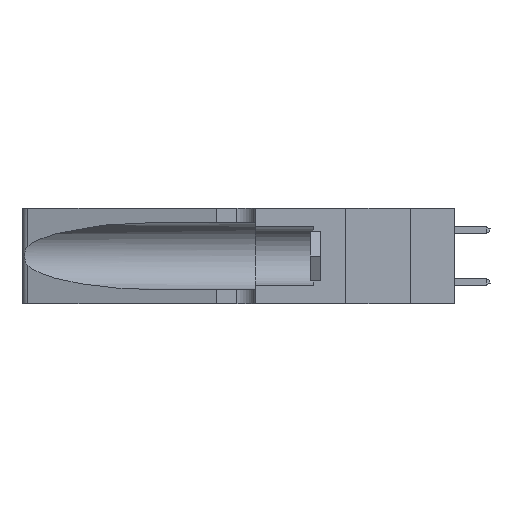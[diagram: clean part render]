
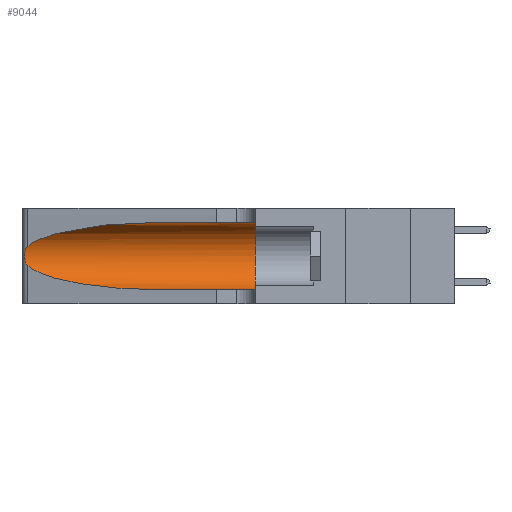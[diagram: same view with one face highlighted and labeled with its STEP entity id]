
A CAD part, left-side view. The second image highlights one B-rep face of the part: STEP entity #9044.
In plain terms, the highlighted cylindrical face has radius 3.308 mm (diameter 6.617 mm), a partial arc.
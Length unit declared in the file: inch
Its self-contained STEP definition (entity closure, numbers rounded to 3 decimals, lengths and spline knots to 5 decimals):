
#729 = VERTEX_POINT ( 'NONE', #15652 ) ;
#792 = EDGE_CURVE ( 'NONE', #729, #7416, #15196, .T. ) ;
#983 = CARTESIAN_POINT ( 'NONE',  ( 0.1305, 0.35, 0.31525 ) ) ;
#1715 = CARTESIAN_POINT ( 'NONE',  ( 0.1305, 0.35, 0.185 ) ) ;
#2022 = CARTESIAN_POINT ( 'NONE',  ( 0.1305, 1.61858, 0.185 ) ) ;
#2512 = VECTOR ( 'NONE', #16649, 39.37008 ) ;
#3192 = CARTESIAN_POINT ( 'NONE',  ( 0.2373, 1.15595, 0.28018 ) ) ;
#3324 = CARTESIAN_POINT ( 'NONE',  ( 0.25487, 1.22718, 0.14631 ) ) ;
#3396 = VERTEX_POINT ( 'NONE', #24382 ) ;
#3710 = DIRECTION ( 'NONE',  ( 0., 0., 1. ) ) ;
#4066 = ORIENTED_EDGE ( 'NONE', *, *, #13687, .F. ) ;
#4930 = CARTESIAN_POINT ( 'NONE',  ( 0.1305, 0.72297, 0.05475 ) ) ;
#5242 = EDGE_CURVE ( 'NONE', #3396, #14820, #7758, .T. ) ;
#5308 = CARTESIAN_POINT ( 'NONE',  ( 0.2373, 1.15595, 0.08982 ) ) ;
#6062 = EDGE_CURVE ( 'NONE', #10185, #8558, #24668, .T. ) ;
#6814 = AXIS2_PLACEMENT_3D ( 'NONE', #2022, #19379, #11790 ) ;
#7270 = CARTESIAN_POINT ( 'NONE',  ( 0.18966, 0.96281, 0.05475 ) ) ;
#7416 = VERTEX_POINT ( 'NONE', #22352 ) ;
#7457 = EDGE_CURVE ( 'NONE', #7416, #10185, #17749, .T. ) ;
#7758 = LINE ( 'NONE', #22335, #2512 ) ;
#8362 = CIRCLE ( 'NONE', #15573, 0.13025 ) ;
#8558 = VERTEX_POINT ( 'NONE', #19965 ) ;
#8609 = CARTESIAN_POINT ( 'NONE',  ( 0.25787, 1.23484, 0.2124 ) ) ;
#9044 = ADVANCED_FACE ( 'NONE', ( #18279 ), #17682, .F. ) ;
#9246 = ORIENTED_EDGE ( 'NONE', *, *, #22004, .T. ) ;
#10185 = VERTEX_POINT ( 'NONE', #4930 ) ;
#10332 = CARTESIAN_POINT ( 'NONE',  ( 0.25854, 1.2359, 0.20912 ) ) ;
#10979 = CARTESIAN_POINT ( 'NONE',  ( 0.26018, 1.23835, 0.19895 ) ) ;
#10995 = CARTESIAN_POINT ( 'NONE',  ( 0.26075, 1.23896, 0.19203 ) ) ;
#11029 = CARTESIAN_POINT ( 'NONE',  ( 0.26075, 1.23896, 0.178 ) ) ;
#11055 = CARTESIAN_POINT ( 'NONE',  ( 0.26017, 1.23833, 0.17102 ) ) ;
#11076 = CARTESIAN_POINT ( 'NONE',  ( 0.25856, 1.23593, 0.16098 ) ) ;
#11104 = ORIENTED_EDGE ( 'NONE', *, *, #5242, .F. ) ;
#11790 = DIRECTION ( 'NONE',  ( 0., 0., -1. ) ) ;
#12832 = CARTESIAN_POINT ( 'NONE',  ( 0.18966, 0.96281, 0.31525 ) ) ;
#13687 = EDGE_CURVE ( 'NONE', #14820, #8558, #8362, .T. ) ;
#14029 = CARTESIAN_POINT ( 'NONE',  ( 0.25555, 1.22994, 0.2215 ) ) ;
#14566 = DIRECTION ( 'NONE',  ( 0., -1., 0. ) ) ;
#14820 = VERTEX_POINT ( 'NONE', #983 ) ;
#15196 = B_SPLINE_CURVE_WITH_KNOTS ( 'NONE', 3,
 ( #20572, #14029, #21229, #8609, #10332, #10979, #10995, #11029, #11055, #11076, #23050, #23037, #17656, #21944 ),
 .UNSPECIFIED., .F., .F.,
 ( 4, 2, 2, 2, 2, 2, 4 ),
 ( 0., 0.00027, 0.00053, 0.00107, 0.0016, 0.00187, 0.00214 ),
 .UNSPECIFIED. ) ;
#15281 = DIRECTION ( 'NONE',  ( 0., 1., 0. ) ) ;
#15573 = AXIS2_PLACEMENT_3D ( 'NONE', #1715, #15281, #3710 ) ;
#15652 = CARTESIAN_POINT ( 'NONE',  ( 0.25487, 1.22718, 0.22369 ) ) ;
#16430 = ORIENTED_EDGE ( 'NONE', *, *, #6062, .T. ) ;
#16649 = DIRECTION ( 'NONE',  ( 0., -1., 0. ) ) ;
#16705 = CARTESIAN_POINT ( 'NONE',  ( 0.25487, 1.22718, 0.22369 ) ) ;
#17656 = CARTESIAN_POINT ( 'NONE',  ( 0.25555, 1.22993, 0.14849 ) ) ;
#17682 = CYLINDRICAL_SURFACE ( 'NONE', #6814, 0.13025 ) ;
#17749 =( BOUNDED_CURVE ( )  B_SPLINE_CURVE ( 3, ( #3324, #5308, #7270, #20599 ),
 .UNSPECIFIED., .F., .T. ) 
 B_SPLINE_CURVE_WITH_KNOTS ( ( 4, 4 ),
 ( 3.44316, 4.71239 ),
 .UNSPECIFIED. ) 
 CURVE ( )  GEOMETRIC_REPRESENTATION_ITEM ( )  RATIONAL_B_SPLINE_CURVE ( ( 1., 0.87, 0.87, 1. ) ) 
 REPRESENTATION_ITEM ( '' )  );
#18279 = FACE_OUTER_BOUND ( 'NONE', #18782, .T. ) ;
#18782 = EDGE_LOOP ( 'NONE', ( #9246, #23789, #24384, #16430, #4066, #11104 ) ) ;
#19379 = DIRECTION ( 'NONE',  ( 0., -1., 0. ) ) ;
#19624 = VECTOR ( 'NONE', #14566, 39.37008 ) ;
#19965 = CARTESIAN_POINT ( 'NONE',  ( 0.1305, 0.35, 0.05475 ) ) ;
#20154 = CARTESIAN_POINT ( 'NONE',  ( 0.1305, 1.61858, 0.05475 ) ) ;
#20572 = CARTESIAN_POINT ( 'NONE',  ( 0.25487, 1.22718, 0.22369 ) ) ;
#20599 = CARTESIAN_POINT ( 'NONE',  ( 0.1305, 0.72297, 0.05475 ) ) ;
#21229 = CARTESIAN_POINT ( 'NONE',  ( 0.25639, 1.23184, 0.21858 ) ) ;
#21944 = CARTESIAN_POINT ( 'NONE',  ( 0.25487, 1.22718, 0.14631 ) ) ;
#22004 = EDGE_CURVE ( 'NONE', #3396, #729, #24730, .T. ) ;
#22335 = CARTESIAN_POINT ( 'NONE',  ( 0.1305, 1.61858, 0.31525 ) ) ;
#22352 = CARTESIAN_POINT ( 'NONE',  ( 0.25487, 1.22718, 0.14631 ) ) ;
#23037 = CARTESIAN_POINT ( 'NONE',  ( 0.25639, 1.23186, 0.15144 ) ) ;
#23050 = CARTESIAN_POINT ( 'NONE',  ( 0.25789, 1.23486, 0.15765 ) ) ;
#23789 = ORIENTED_EDGE ( 'NONE', *, *, #792, .T. ) ;
#24202 = CARTESIAN_POINT ( 'NONE',  ( 0.1305, 0.72297, 0.31525 ) ) ;
#24382 = CARTESIAN_POINT ( 'NONE',  ( 0.1305, 0.72297, 0.31525 ) ) ;
#24384 = ORIENTED_EDGE ( 'NONE', *, *, #7457, .T. ) ;
#24668 = LINE ( 'NONE', #20154, #19624 ) ;
#24730 =( BOUNDED_CURVE ( )  B_SPLINE_CURVE ( 3, ( #24202, #12832, #3192, #16705 ),
 .UNSPECIFIED., .F., .F. ) 
 B_SPLINE_CURVE_WITH_KNOTS ( ( 4, 4 ),
 ( 1.5708, 2.84003 ),
 .UNSPECIFIED. ) 
 CURVE ( )  GEOMETRIC_REPRESENTATION_ITEM ( )  RATIONAL_B_SPLINE_CURVE ( ( 1., 0.87, 0.87, 1. ) ) 
 REPRESENTATION_ITEM ( '' )  );
